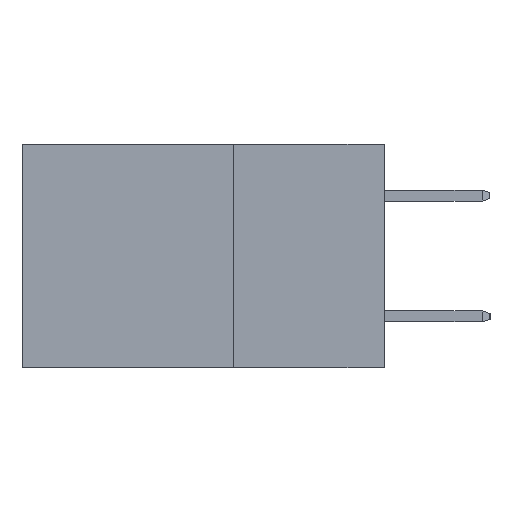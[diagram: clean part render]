
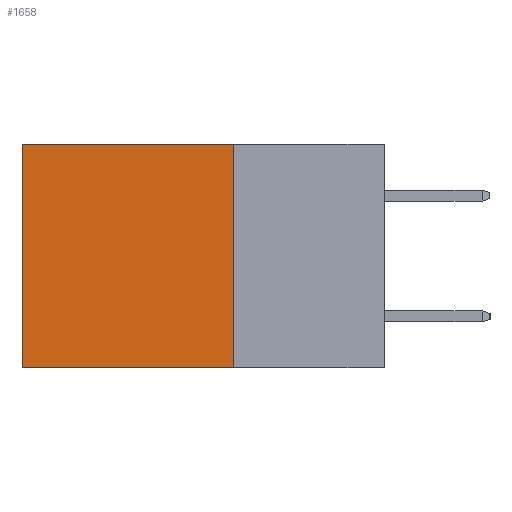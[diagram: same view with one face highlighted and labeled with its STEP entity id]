
A CAD part, left-side view. The second image highlights one B-rep face of the part: STEP entity #1658.
In plain terms, the highlighted planar face has unit normal (-1, 0, 0).
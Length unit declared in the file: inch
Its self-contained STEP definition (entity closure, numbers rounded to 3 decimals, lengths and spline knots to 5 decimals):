
#170 = DIRECTION ( 'NONE',  ( 0., 1., 0. ) ) ;
#511 = ORIENTED_EDGE ( 'NONE', *, *, #5706, .F. ) ;
#542 = CARTESIAN_POINT ( 'NONE',  ( 0.2615, 0.25, -0.37 ) ) ;
#690 = ORIENTED_EDGE ( 'NONE', *, *, #3812, .T. ) ;
#1658 = ADVANCED_FACE ( 'NONE', ( #10265 ), #2698, .F. ) ;
#1786 = CARTESIAN_POINT ( 'NONE',  ( 0.2615, 0.6, -0.37 ) ) ;
#2042 = AXIS2_PLACEMENT_3D ( 'NONE', #3655, #4591, #10942 ) ;
#2281 = LINE ( 'NONE', #542, #7256 ) ;
#2698 = PLANE ( 'NONE',  #2042 ) ;
#3541 = VERTEX_POINT ( 'NONE', #6208 ) ;
#3595 = VERTEX_POINT ( 'NONE', #5352 ) ;
#3620 = EDGE_LOOP ( 'NONE', ( #9360, #511, #10930, #690 ) ) ;
#3655 = CARTESIAN_POINT ( 'NONE',  ( 0.2615, 0.25, -0.37 ) ) ;
#3812 = EDGE_CURVE ( 'NONE', #4200, #3541, #9960, .T. ) ;
#4200 = VERTEX_POINT ( 'NONE', #5139 ) ;
#4571 = DIRECTION ( 'NONE',  ( 0., 0., -1. ) ) ;
#4591 = DIRECTION ( 'NONE',  ( 1., 0., 0. ) ) ;
#4650 = VERTEX_POINT ( 'NONE', #8434 ) ;
#5139 = CARTESIAN_POINT ( 'NONE',  ( 0.2615, 0.25, 0. ) ) ;
#5227 = EDGE_CURVE ( 'NONE', #3541, #3595, #9648, .T. ) ;
#5352 = CARTESIAN_POINT ( 'NONE',  ( 0.2615, 0.6, -0.37 ) ) ;
#5706 = EDGE_CURVE ( 'NONE', #4650, #3595, #2281, .T. ) ;
#6208 = CARTESIAN_POINT ( 'NONE',  ( 0.2615, 0.6, 0. ) ) ;
#6915 = LINE ( 'NONE', #9835, #11106 ) ;
#7256 = VECTOR ( 'NONE', #11580, 39.37008 ) ;
#7269 = VECTOR ( 'NONE', #4571, 39.37008 ) ;
#8434 = CARTESIAN_POINT ( 'NONE',  ( 0.2615, 0.25, -0.37 ) ) ;
#9360 = ORIENTED_EDGE ( 'NONE', *, *, #5227, .T. ) ;
#9648 = LINE ( 'NONE', #1786, #7269 ) ;
#9684 = VECTOR ( 'NONE', #170, 39.37008 ) ;
#9835 = CARTESIAN_POINT ( 'NONE',  ( 0.2615, 0.25, -0.37 ) ) ;
#9856 = EDGE_CURVE ( 'NONE', #4200, #4650, #6915, .T. ) ;
#9960 = LINE ( 'NONE', #11169, #9684 ) ;
#10265 = FACE_OUTER_BOUND ( 'NONE', #3620, .T. ) ;
#10930 = ORIENTED_EDGE ( 'NONE', *, *, #9856, .F. ) ;
#10942 = DIRECTION ( 'NONE',  ( 0., 0., -1. ) ) ;
#11106 = VECTOR ( 'NONE', #11614, 39.37008 ) ;
#11169 = CARTESIAN_POINT ( 'NONE',  ( 0.2615, 0.25, 0. ) ) ;
#11580 = DIRECTION ( 'NONE',  ( 0., 1., 0. ) ) ;
#11614 = DIRECTION ( 'NONE',  ( 0., 0., -1. ) ) ;
